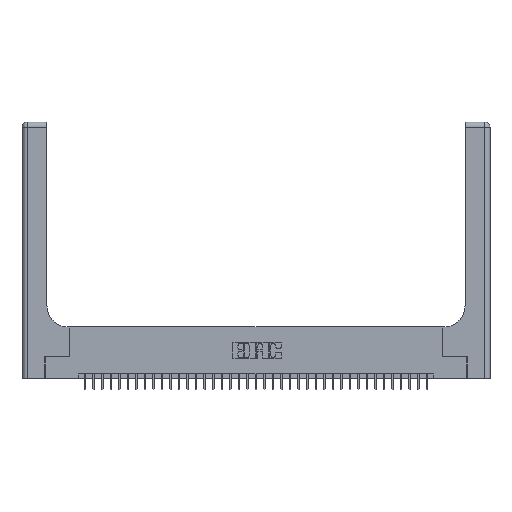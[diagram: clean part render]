
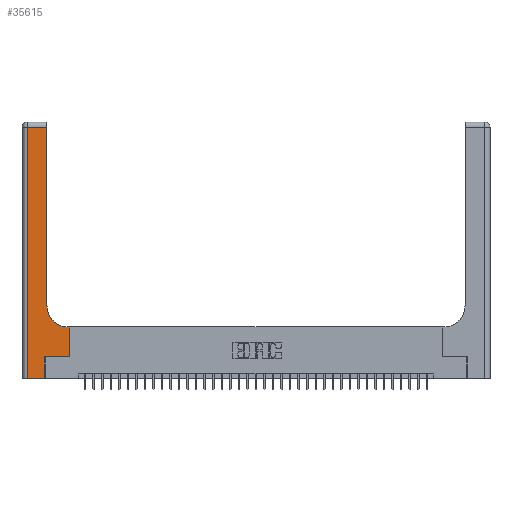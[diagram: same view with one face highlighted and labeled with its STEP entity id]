
A CAD part, top view. The second image highlights one B-rep face of the part: STEP entity #35615.
In plain terms, the highlighted planar face has unit normal (0, 0, 1).
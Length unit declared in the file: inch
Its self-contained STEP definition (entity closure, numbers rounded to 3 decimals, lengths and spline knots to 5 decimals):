
#2342 = CARTESIAN_POINT ( 'NONE',  ( 0.2915, 2.94, 0.37 ) ) ;
#2586 = EDGE_CURVE ( 'NONE', #8839, #20168, #10718, .T. ) ;
#2842 = CIRCLE ( 'NONE', #25926, 0.25 ) ;
#2978 = CARTESIAN_POINT ( 'NONE',  ( 0.2915, 0.6, 0.37 ) ) ;
#4476 = CARTESIAN_POINT ( 'NONE',  ( 0.269, 0.25, 0.37 ) ) ;
#4879 = EDGE_CURVE ( 'NONE', #37516, #30963, #19217, .T. ) ;
#6133 = VERTEX_POINT ( 'NONE', #28171 ) ;
#6694 = EDGE_CURVE ( 'NONE', #6133, #30589, #20114, .T. ) ;
#7466 = VERTEX_POINT ( 'NONE', #30069 ) ;
#7496 = ORIENTED_EDGE ( 'NONE', *, *, #19006, .T. ) ;
#8403 = CARTESIAN_POINT ( 'NONE',  ( 0.2915, 0.85, 0.37 ) ) ;
#8669 = DIRECTION ( 'NONE',  ( -1., 0., 0. ) ) ;
#8839 = VERTEX_POINT ( 'NONE', #26683 ) ;
#9021 = ORIENTED_EDGE ( 'NONE', *, *, #15969, .T. ) ;
#9531 = LINE ( 'NONE', #33127, #23890 ) ;
#9833 = DIRECTION ( 'NONE',  ( 0., 1., 0. ) ) ;
#10718 = LINE ( 'NONE', #27485, #21995 ) ;
#10952 = VECTOR ( 'NONE', #36377, 39.37008 ) ;
#11185 = EDGE_CURVE ( 'NONE', #20168, #7466, #15325, .T. ) ;
#12574 = DIRECTION ( 'NONE',  ( 0., -1., 0. ) ) ;
#12629 = VECTOR ( 'NONE', #8669, 39.37008 ) ;
#12694 = CARTESIAN_POINT ( 'NONE',  ( 0.2915, 3., 0.37 ) ) ;
#13103 = DIRECTION ( 'NONE',  ( 1., 0., 0. ) ) ;
#13351 = CARTESIAN_POINT ( 'NONE',  ( 0., 2.94, 0.37 ) ) ;
#14608 = DIRECTION ( 'NONE',  ( 0., 1., 0. ) ) ;
#14772 = VECTOR ( 'NONE', #13103, 39.37008 ) ;
#15325 = LINE ( 'NONE', #2978, #12629 ) ;
#15677 = VECTOR ( 'NONE', #14608, 39.37008 ) ;
#15969 = EDGE_CURVE ( 'NONE', #30589, #8839, #27788, .T. ) ;
#16301 = DIRECTION ( 'NONE',  ( 0., 0., -1. ) ) ;
#16542 = CARTESIAN_POINT ( 'NONE',  ( 0.269, 0.25, 0.37 ) ) ;
#18491 = EDGE_LOOP ( 'NONE', ( #26386, #26247, #7496, #22169, #31672, #9021, #34891, #34301, #22508 ) ) ;
#19006 = EDGE_CURVE ( 'NONE', #30963, #21283, #9531, .T. ) ;
#19141 = CARTESIAN_POINT ( 'NONE',  ( 0.5415, 0.85, 0.37 ) ) ;
#19217 = LINE ( 'NONE', #13351, #27249 ) ;
#19657 = DIRECTION ( 'NONE',  ( -1., 0., 0. ) ) ;
#19844 = PLANE ( 'NONE',  #26034 ) ;
#20114 = LINE ( 'NONE', #31346, #15677 ) ;
#20168 = VERTEX_POINT ( 'NONE', #32225 ) ;
#21283 = VERTEX_POINT ( 'NONE', #37123 ) ;
#21959 = DIRECTION ( 'NONE',  ( 0., 1., 0. ) ) ;
#21995 = VECTOR ( 'NONE', #21959, 39.37008 ) ;
#22169 = ORIENTED_EDGE ( 'NONE', *, *, #27281, .T. ) ;
#22508 = ORIENTED_EDGE ( 'NONE', *, *, #33641, .T. ) ;
#22898 = FACE_OUTER_BOUND ( 'NONE', #18491, .T. ) ;
#23890 = VECTOR ( 'NONE', #12574, 39.37008 ) ;
#25765 = DIRECTION ( 'NONE',  ( 0., 0., -1. ) ) ;
#25926 = AXIS2_PLACEMENT_3D ( 'NONE', #19141, #16301, #33261 ) ;
#26034 = AXIS2_PLACEMENT_3D ( 'NONE', #31651, #25765, #19657 ) ;
#26247 = ORIENTED_EDGE ( 'NONE', *, *, #4879, .T. ) ;
#26386 = ORIENTED_EDGE ( 'NONE', *, *, #28846, .T. ) ;
#26683 = CARTESIAN_POINT ( 'NONE',  ( 0.5585, 0.25, 0.37 ) ) ;
#26879 = CARTESIAN_POINT ( 'NONE',  ( 0.06, 2.94, 0.37 ) ) ;
#27249 = VECTOR ( 'NONE', #34072, 39.37008 ) ;
#27281 = EDGE_CURVE ( 'NONE', #21283, #6133, #28286, .T. ) ;
#27485 = CARTESIAN_POINT ( 'NONE',  ( 0.5585, 0.25, 0.37 ) ) ;
#27788 = LINE ( 'NONE', #16542, #10952 ) ;
#28171 = CARTESIAN_POINT ( 'NONE',  ( 0.269, 0., 0.37 ) ) ;
#28286 = LINE ( 'NONE', #37058, #14772 ) ;
#28846 = EDGE_CURVE ( 'NONE', #36067, #37516, #30379, .T. ) ;
#30069 = CARTESIAN_POINT ( 'NONE',  ( 0.5415, 0.6, 0.37 ) ) ;
#30379 = LINE ( 'NONE', #12694, #31846 ) ;
#30589 = VERTEX_POINT ( 'NONE', #4476 ) ;
#30963 = VERTEX_POINT ( 'NONE', #26879 ) ;
#31346 = CARTESIAN_POINT ( 'NONE',  ( 0.269, 0., 0.37 ) ) ;
#31651 = CARTESIAN_POINT ( 'NONE',  ( 0., 3., 0.37 ) ) ;
#31672 = ORIENTED_EDGE ( 'NONE', *, *, #6694, .T. ) ;
#31846 = VECTOR ( 'NONE', #9833, 39.37008 ) ;
#32225 = CARTESIAN_POINT ( 'NONE',  ( 0.5585, 0.6, 0.37 ) ) ;
#33127 = CARTESIAN_POINT ( 'NONE',  ( 0.06, 3., 0.37 ) ) ;
#33261 = DIRECTION ( 'NONE',  ( 1., 0., 0. ) ) ;
#33641 = EDGE_CURVE ( 'NONE', #7466, #36067, #2842, .T. ) ;
#34072 = DIRECTION ( 'NONE',  ( -1., 0., 0. ) ) ;
#34301 = ORIENTED_EDGE ( 'NONE', *, *, #11185, .T. ) ;
#34891 = ORIENTED_EDGE ( 'NONE', *, *, #2586, .T. ) ;
#35615 = ADVANCED_FACE ( 'NONE', ( #22898 ), #19844, .F. ) ;
#36067 = VERTEX_POINT ( 'NONE', #8403 ) ;
#36377 = DIRECTION ( 'NONE',  ( 1., 0., 0. ) ) ;
#37058 = CARTESIAN_POINT ( 'NONE',  ( 0., 0., 0.37 ) ) ;
#37123 = CARTESIAN_POINT ( 'NONE',  ( 0.06, 0., 0.37 ) ) ;
#37516 = VERTEX_POINT ( 'NONE', #2342 ) ;
